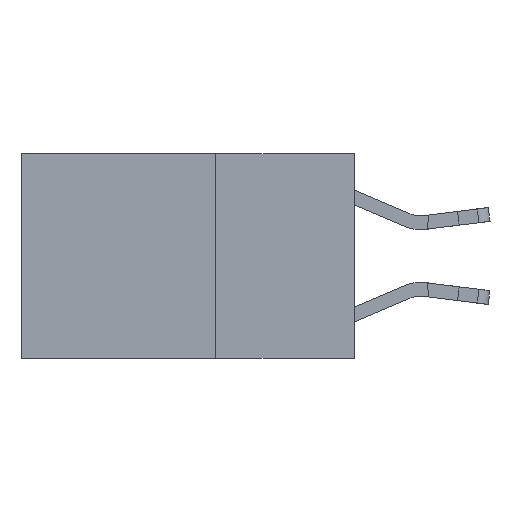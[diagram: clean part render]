
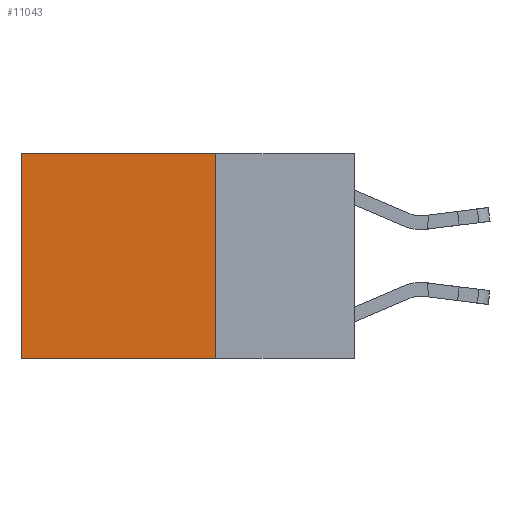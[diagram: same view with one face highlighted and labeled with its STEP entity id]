
A CAD part, left-side view. The second image highlights one B-rep face of the part: STEP entity #11043.
In plain terms, the highlighted planar face has unit normal (-1, 0, 0).
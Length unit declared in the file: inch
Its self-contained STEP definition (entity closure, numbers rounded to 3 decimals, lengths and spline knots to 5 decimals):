
#76 = ORIENTED_EDGE ( 'NONE', *, *, #8219, .T. ) ;
#1056 = VERTEX_POINT ( 'NONE', #2781 ) ;
#1087 = CARTESIAN_POINT ( 'NONE',  ( 0.2625, 0.6, 0. ) ) ;
#1436 = EDGE_LOOP ( 'NONE', ( #76, #8146, #10363, #6103 ) ) ;
#1840 = EDGE_CURVE ( 'NONE', #9640, #5499, #9519, .T. ) ;
#1944 = CARTESIAN_POINT ( 'NONE',  ( 0.2625, 0.6, -0.37 ) ) ;
#2062 = CARTESIAN_POINT ( 'NONE',  ( 0.2625, 0.25, 0. ) ) ;
#2582 = VECTOR ( 'NONE', #13335, 39.37008 ) ;
#2781 = CARTESIAN_POINT ( 'NONE',  ( 0.2625, 0.25, 0. ) ) ;
#3916 = AXIS2_PLACEMENT_3D ( 'NONE', #2062, #6567, #10991 ) ;
#3964 = LINE ( 'NONE', #4997, #4325 ) ;
#4280 = CARTESIAN_POINT ( 'NONE',  ( 0.2625, 0.25, -0.37 ) ) ;
#4325 = VECTOR ( 'NONE', #13864, 39.37008 ) ;
#4429 = CARTESIAN_POINT ( 'NONE',  ( 0.2625, 0.25, 0. ) ) ;
#4997 = CARTESIAN_POINT ( 'NONE',  ( 0.2625, 0.25, 0. ) ) ;
#5150 = CARTESIAN_POINT ( 'NONE',  ( 0.2625, 0.25, -0.37 ) ) ;
#5499 = VERTEX_POINT ( 'NONE', #1944 ) ;
#5529 = FACE_OUTER_BOUND ( 'NONE', #1436, .T. ) ;
#6043 = VECTOR ( 'NONE', #6665, 39.37008 ) ;
#6103 = ORIENTED_EDGE ( 'NONE', *, *, #14125, .T. ) ;
#6294 = VECTOR ( 'NONE', #12806, 39.37008 ) ;
#6567 = DIRECTION ( 'NONE',  ( 1., 0., 0. ) ) ;
#6665 = DIRECTION ( 'NONE',  ( 0., 0., -1. ) ) ;
#7816 = CARTESIAN_POINT ( 'NONE',  ( 0.2625, 0.6, 0. ) ) ;
#8146 = ORIENTED_EDGE ( 'NONE', *, *, #1840, .F. ) ;
#8219 = EDGE_CURVE ( 'NONE', #11947, #5499, #11293, .T. ) ;
#8845 = EDGE_CURVE ( 'NONE', #1056, #9640, #3964, .T. ) ;
#9192 = LINE ( 'NONE', #4429, #2582 ) ;
#9519 = LINE ( 'NONE', #5150, #6294 ) ;
#9640 = VERTEX_POINT ( 'NONE', #4280 ) ;
#10363 = ORIENTED_EDGE ( 'NONE', *, *, #8845, .F. ) ;
#10991 = DIRECTION ( 'NONE',  ( 0., 0., -1. ) ) ;
#11043 = ADVANCED_FACE ( 'NONE', ( #5529 ), #14028, .F. ) ;
#11293 = LINE ( 'NONE', #7816, #6043 ) ;
#11947 = VERTEX_POINT ( 'NONE', #1087 ) ;
#12806 = DIRECTION ( 'NONE',  ( 0., 1., 0. ) ) ;
#13335 = DIRECTION ( 'NONE',  ( 0., 1., 0. ) ) ;
#13864 = DIRECTION ( 'NONE',  ( 0., 0., -1. ) ) ;
#14028 = PLANE ( 'NONE',  #3916 ) ;
#14125 = EDGE_CURVE ( 'NONE', #1056, #11947, #9192, .T. ) ;
